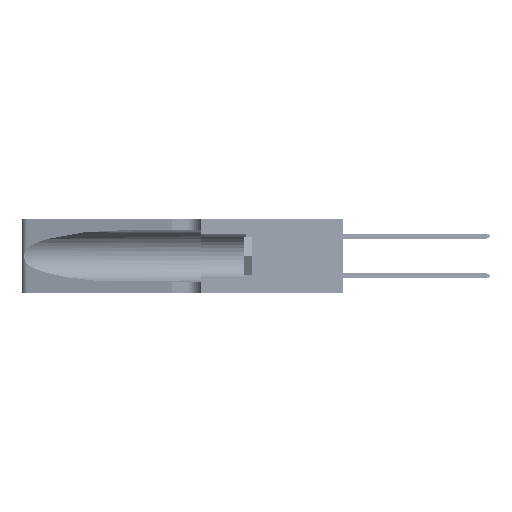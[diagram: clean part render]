
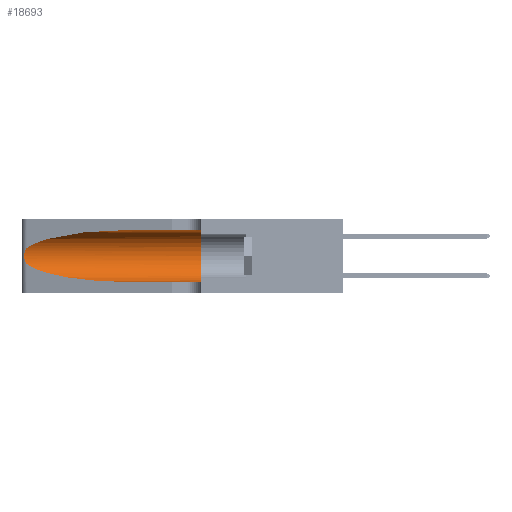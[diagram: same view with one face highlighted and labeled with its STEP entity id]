
A CAD part, left-side view. The second image highlights one B-rep face of the part: STEP entity #18693.
In plain terms, the highlighted cylindrical face has radius 3.308 mm (diameter 6.617 mm), a partial arc.
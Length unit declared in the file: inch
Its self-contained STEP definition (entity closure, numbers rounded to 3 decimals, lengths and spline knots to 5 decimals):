
#1945 = CARTESIAN_POINT ( 'NONE',  ( 0.26017, 1.23833, 0.17102 ) ) ;
#2514 = EDGE_CURVE ( 'NONE', #43194, #43030, #44906, .T. ) ;
#3433 = CARTESIAN_POINT ( 'NONE',  ( 0.25487, 1.22718, 0.22369 ) ) ;
#5027 = ORIENTED_EDGE ( 'NONE', *, *, #34445, .F. ) ;
#5081 = CARTESIAN_POINT ( 'NONE',  ( 0.25487, 1.22718, 0.22369 ) ) ;
#5240 = CARTESIAN_POINT ( 'NONE',  ( 0.25639, 1.23186, 0.15144 ) ) ;
#6753 = VERTEX_POINT ( 'NONE', #23207 ) ;
#7300 = VERTEX_POINT ( 'NONE', #26990 ) ;
#8088 = ORIENTED_EDGE ( 'NONE', *, *, #11683, .F. ) ;
#8195 = CARTESIAN_POINT ( 'NONE',  ( 0.25787, 1.23484, 0.2124 ) ) ;
#8791 = CARTESIAN_POINT ( 'NONE',  ( 0.1305, 1.61858, 0.05475 ) ) ;
#11544 = DIRECTION ( 'NONE',  ( 0., -1., 0. ) ) ;
#11683 = EDGE_CURVE ( 'NONE', #6753, #19242, #48935, .T. ) ;
#12197 = CARTESIAN_POINT ( 'NONE',  ( 0.26018, 1.23835, 0.19895 ) ) ;
#14066 = CARTESIAN_POINT ( 'NONE',  ( 0.2373, 1.15595, 0.28018 ) ) ;
#15609 = CARTESIAN_POINT ( 'NONE',  ( 0.1305, 0.72297, 0.05475 ) ) ;
#16222 = CARTESIAN_POINT ( 'NONE',  ( 0.26075, 1.23896, 0.178 ) ) ;
#16233 = CARTESIAN_POINT ( 'NONE',  ( 0.1305, 0.35, 0.185 ) ) ;
#18427 = AXIS2_PLACEMENT_3D ( 'NONE', #19753, #11544, #47048 ) ;
#18606 = CARTESIAN_POINT ( 'NONE',  ( 0.1305, 0.72297, 0.31525 ) ) ;
#18693 = ADVANCED_FACE ( 'NONE', ( #40410 ), #31106, .F. ) ;
#19242 = VERTEX_POINT ( 'NONE', #30118 ) ;
#19753 = CARTESIAN_POINT ( 'NONE',  ( 0.1305, 1.61858, 0.185 ) ) ;
#20375 = B_SPLINE_CURVE_WITH_KNOTS ( 'NONE', 3,
 ( #5081, #24703, #48707, #8195, #35991, #12197, #40004, #16222, #1945, #45546, #29056, #5240, #29735, #33380 ),
 .UNSPECIFIED., .F., .F.,
 ( 4, 2, 2, 2, 2, 2, 4 ),
 ( 0., 0.00027, 0.00053, 0.00107, 0.0016, 0.00187, 0.00214 ),
 .UNSPECIFIED. ) ;
#20553 = VECTOR ( 'NONE', #27599, 39.37008 ) ;
#21462 = ORIENTED_EDGE ( 'NONE', *, *, #25954, .T. ) ;
#23207 = CARTESIAN_POINT ( 'NONE',  ( 0.1305, 0.35, 0.31525 ) ) ;
#23987 = ORIENTED_EDGE ( 'NONE', *, *, #43093, .T. ) ;
#24029 = EDGE_CURVE ( 'NONE', #43030, #43887, #20375, .T. ) ;
#24616 = DIRECTION ( 'NONE',  ( 0., -1., 0. ) ) ;
#24703 = CARTESIAN_POINT ( 'NONE',  ( 0.25555, 1.22994, 0.2215 ) ) ;
#24874 = AXIS2_PLACEMENT_3D ( 'NONE', #16233, #48720, #28196 ) ;
#25954 = EDGE_CURVE ( 'NONE', #7300, #19242, #42032, .T. ) ;
#26065 = CARTESIAN_POINT ( 'NONE',  ( 0.25487, 1.22718, 0.22369 ) ) ;
#26990 = CARTESIAN_POINT ( 'NONE',  ( 0.1305, 0.72297, 0.05475 ) ) ;
#27599 = DIRECTION ( 'NONE',  ( 0., -1., 0. ) ) ;
#28196 = DIRECTION ( 'NONE',  ( 0., 0., 1. ) ) ;
#29056 = CARTESIAN_POINT ( 'NONE',  ( 0.25789, 1.23486, 0.15765 ) ) ;
#29735 = CARTESIAN_POINT ( 'NONE',  ( 0.25555, 1.22993, 0.14849 ) ) ;
#30118 = CARTESIAN_POINT ( 'NONE',  ( 0.1305, 0.35, 0.05475 ) ) ;
#30521 = LINE ( 'NONE', #39064, #20553 ) ;
#31106 = CYLINDRICAL_SURFACE ( 'NONE', #18427, 0.13025 ) ;
#31233 = CARTESIAN_POINT ( 'NONE',  ( 0.18966, 0.96281, 0.05475 ) ) ;
#31473 = VECTOR ( 'NONE', #24616, 39.37008 ) ;
#33380 = CARTESIAN_POINT ( 'NONE',  ( 0.25487, 1.22718, 0.14631 ) ) ;
#34198 = CARTESIAN_POINT ( 'NONE',  ( 0.18966, 0.96281, 0.31525 ) ) ;
#34445 = EDGE_CURVE ( 'NONE', #43194, #6753, #30521, .T. ) ;
#34794 = EDGE_LOOP ( 'NONE', ( #49091, #39127, #23987, #21462, #8088, #5027 ) ) ;
#35562 = CARTESIAN_POINT ( 'NONE',  ( 0.2373, 1.15595, 0.08982 ) ) ;
#35991 = CARTESIAN_POINT ( 'NONE',  ( 0.25854, 1.2359, 0.20912 ) ) ;
#39064 = CARTESIAN_POINT ( 'NONE',  ( 0.1305, 1.61858, 0.31525 ) ) ;
#39127 = ORIENTED_EDGE ( 'NONE', *, *, #24029, .T. ) ;
#40004 = CARTESIAN_POINT ( 'NONE',  ( 0.26075, 1.23896, 0.19203 ) ) ;
#40173 = CARTESIAN_POINT ( 'NONE',  ( 0.25487, 1.22718, 0.14631 ) ) ;
#40402 = CARTESIAN_POINT ( 'NONE',  ( 0.1305, 0.72297, 0.31525 ) ) ;
#40410 = FACE_OUTER_BOUND ( 'NONE', #34794, .T. ) ;
#42032 = LINE ( 'NONE', #8791, #31473 ) ;
#43030 = VERTEX_POINT ( 'NONE', #3433 ) ;
#43093 = EDGE_CURVE ( 'NONE', #43887, #7300, #50361, .T. ) ;
#43194 = VERTEX_POINT ( 'NONE', #40402 ) ;
#43887 = VERTEX_POINT ( 'NONE', #40173 ) ;
#44906 =( BOUNDED_CURVE ( )  B_SPLINE_CURVE ( 3, ( #18606, #34198, #14066, #26065 ),
 .UNSPECIFIED., .F., .F. ) 
 B_SPLINE_CURVE_WITH_KNOTS ( ( 4, 4 ),
 ( 1.5708, 2.84003 ),
 .UNSPECIFIED. ) 
 CURVE ( )  GEOMETRIC_REPRESENTATION_ITEM ( )  RATIONAL_B_SPLINE_CURVE ( ( 1., 0.87, 0.87, 1. ) ) 
 REPRESENTATION_ITEM ( '' )  );
#45546 = CARTESIAN_POINT ( 'NONE',  ( 0.25856, 1.23593, 0.16098 ) ) ;
#46909 = CARTESIAN_POINT ( 'NONE',  ( 0.25487, 1.22718, 0.14631 ) ) ;
#47048 = DIRECTION ( 'NONE',  ( 0., 0., -1. ) ) ;
#48707 = CARTESIAN_POINT ( 'NONE',  ( 0.25639, 1.23184, 0.21858 ) ) ;
#48720 = DIRECTION ( 'NONE',  ( 0., 1., 0. ) ) ;
#48935 = CIRCLE ( 'NONE', #24874, 0.13025 ) ;
#49091 = ORIENTED_EDGE ( 'NONE', *, *, #2514, .T. ) ;
#50361 =( BOUNDED_CURVE ( )  B_SPLINE_CURVE ( 3, ( #46909, #35562, #31233, #15609 ),
 .UNSPECIFIED., .F., .F. ) 
 B_SPLINE_CURVE_WITH_KNOTS ( ( 4, 4 ),
 ( 3.44316, 4.71239 ),
 .UNSPECIFIED. ) 
 CURVE ( )  GEOMETRIC_REPRESENTATION_ITEM ( )  RATIONAL_B_SPLINE_CURVE ( ( 1., 0.87, 0.87, 1. ) ) 
 REPRESENTATION_ITEM ( '' )  );
